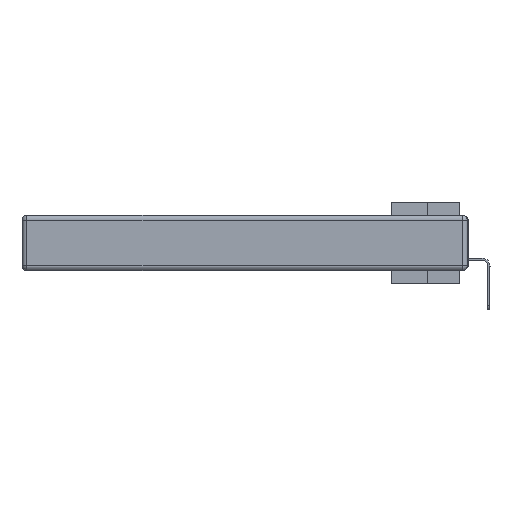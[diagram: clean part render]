
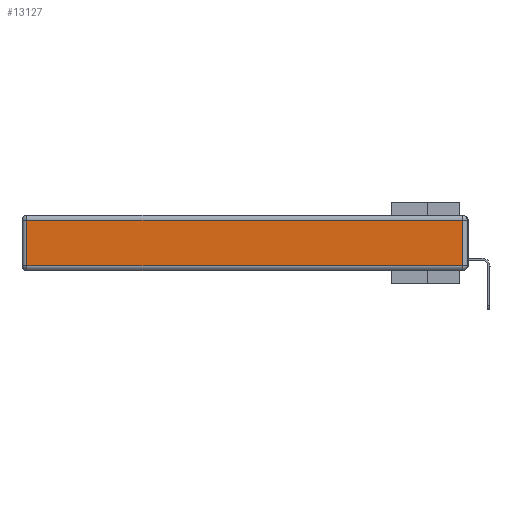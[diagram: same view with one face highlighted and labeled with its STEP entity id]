
A CAD part, left-side view. The second image highlights one B-rep face of the part: STEP entity #13127.
In plain terms, the highlighted planar face has unit normal (-1, 0, 0).
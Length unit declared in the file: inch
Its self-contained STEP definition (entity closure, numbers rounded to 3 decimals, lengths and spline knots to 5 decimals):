
#1788 = DIRECTION ( 'NONE',  ( 0., -1., 0. ) ) ;
#2906 = DIRECTION ( 'NONE',  ( -1., 0., 0. ) ) ;
#3323 = DIRECTION ( 'NONE',  ( 0., 0., 1. ) ) ;
#3742 = VERTEX_POINT ( 'NONE', #27760 ) ;
#4185 = ORIENTED_EDGE ( 'NONE', *, *, #24579, .T. ) ;
#4276 = CARTESIAN_POINT ( 'NONE',  ( 0., 2.75, -0.03 ) ) ;
#6082 = VERTEX_POINT ( 'NONE', #25006 ) ;
#6106 = LINE ( 'NONE', #28886, #19196 ) ;
#6141 = LINE ( 'NONE', #12772, #9315 ) ;
#8434 = CARTESIAN_POINT ( 'NONE',  ( 0., 2.72, -0.03 ) ) ;
#9315 = VECTOR ( 'NONE', #21402, 39.37008 ) ;
#9621 = EDGE_LOOP ( 'NONE', ( #17971, #18832, #19844, #4185 ) ) ;
#10122 = CARTESIAN_POINT ( 'NONE',  ( 0., 0.03, -0.343 ) ) ;
#10425 = VERTEX_POINT ( 'NONE', #26499 ) ;
#11783 = VECTOR ( 'NONE', #28285, 39.37008 ) ;
#11842 = VECTOR ( 'NONE', #13086, 39.37008 ) ;
#12253 = EDGE_CURVE ( 'NONE', #10425, #26945, #25248, .T. ) ;
#12772 = CARTESIAN_POINT ( 'NONE',  ( 0., 2.72, -0.343 ) ) ;
#13086 = DIRECTION ( 'NONE',  ( 0., 1., 0. ) ) ;
#13127 = ADVANCED_FACE ( 'NONE', ( #16359 ), #27710, .T. ) ;
#13356 = EDGE_CURVE ( 'NONE', #3742, #6082, #6106, .T. ) ;
#14168 = CARTESIAN_POINT ( 'NONE',  ( 0., 0., -0.343 ) ) ;
#16359 = FACE_OUTER_BOUND ( 'NONE', #9621, .T. ) ;
#17971 = ORIENTED_EDGE ( 'NONE', *, *, #13356, .T. ) ;
#18832 = ORIENTED_EDGE ( 'NONE', *, *, #24442, .T. ) ;
#19196 = VECTOR ( 'NONE', #1788, 39.37008 ) ;
#19844 = ORIENTED_EDGE ( 'NONE', *, *, #12253, .T. ) ;
#20936 = AXIS2_PLACEMENT_3D ( 'NONE', #14168, #2906, #3323 ) ;
#21402 = DIRECTION ( 'NONE',  ( 0., 0., -1. ) ) ;
#24442 = EDGE_CURVE ( 'NONE', #6082, #10425, #26944, .T. ) ;
#24579 = EDGE_CURVE ( 'NONE', #26945, #3742, #6141, .T. ) ;
#25006 = CARTESIAN_POINT ( 'NONE',  ( 0., 0.03, -0.313 ) ) ;
#25248 = LINE ( 'NONE', #4276, #11842 ) ;
#26499 = CARTESIAN_POINT ( 'NONE',  ( 0., 0.03, -0.03 ) ) ;
#26944 = LINE ( 'NONE', #10122, #11783 ) ;
#26945 = VERTEX_POINT ( 'NONE', #8434 ) ;
#27710 = PLANE ( 'NONE',  #20936 ) ;
#27760 = CARTESIAN_POINT ( 'NONE',  ( 0., 2.72, -0.313 ) ) ;
#28285 = DIRECTION ( 'NONE',  ( 0., 0., 1. ) ) ;
#28886 = CARTESIAN_POINT ( 'NONE',  ( 0., 0., -0.313 ) ) ;
